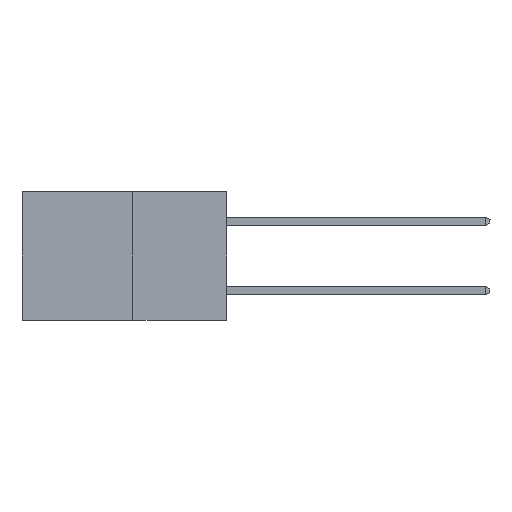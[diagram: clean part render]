
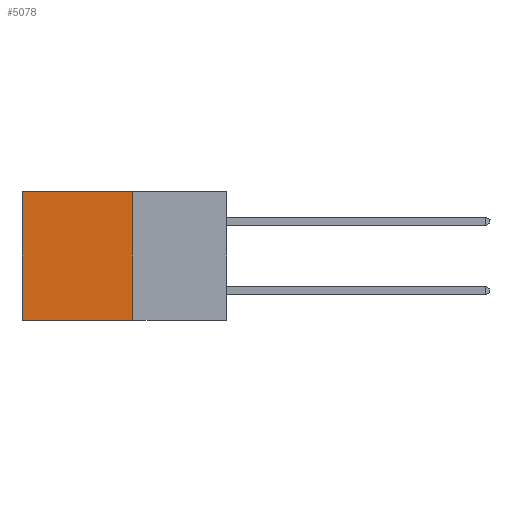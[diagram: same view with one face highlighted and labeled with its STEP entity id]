
A CAD part, left-side view. The second image highlights one B-rep face of the part: STEP entity #5078.
In plain terms, the highlighted planar face has unit normal (-1, 0, 0).
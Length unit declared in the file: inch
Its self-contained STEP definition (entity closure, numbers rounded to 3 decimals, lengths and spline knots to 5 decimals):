
#123 = ORIENTED_EDGE ( 'NONE', *, *, #6466, .T. ) ;
#441 = LINE ( 'NONE', #17034, #2452 ) ;
#500 = DIRECTION ( 'NONE',  ( 0., 1., 0. ) ) ;
#1087 = CARTESIAN_POINT ( 'NONE',  ( 0.277, 0.27, -0.37 ) ) ;
#1097 = VERTEX_POINT ( 'NONE', #2230 ) ;
#1224 = DIRECTION ( 'NONE',  ( 0., 0., -1. ) ) ;
#1623 = LINE ( 'NONE', #4373, #13090 ) ;
#2230 = CARTESIAN_POINT ( 'NONE',  ( 0.277, 0.59, -0.37 ) ) ;
#2452 = VECTOR ( 'NONE', #500, 39.37008 ) ;
#3029 = LINE ( 'NONE', #14663, #14517 ) ;
#4357 = VERTEX_POINT ( 'NONE', #1087 ) ;
#4373 = CARTESIAN_POINT ( 'NONE',  ( 0.277, 0.59, -0.37 ) ) ;
#5078 = ADVANCED_FACE ( 'NONE', ( #9567 ), #16496, .F. ) ;
#6377 = EDGE_CURVE ( 'NONE', #15414, #4357, #3029, .T. ) ;
#6466 = EDGE_CURVE ( 'NONE', #10629, #1097, #1623, .T. ) ;
#6665 = DIRECTION ( 'NONE',  ( 0., 1., 0. ) ) ;
#6745 = EDGE_CURVE ( 'NONE', #15414, #10629, #441, .T. ) ;
#7455 = DIRECTION ( 'NONE',  ( 1., 0., 0. ) ) ;
#8330 = ORIENTED_EDGE ( 'NONE', *, *, #6745, .T. ) ;
#9392 = LINE ( 'NONE', #12560, #12971 ) ;
#9567 = FACE_OUTER_BOUND ( 'NONE', #13771, .T. ) ;
#10029 = EDGE_CURVE ( 'NONE', #4357, #1097, #9392, .T. ) ;
#10629 = VERTEX_POINT ( 'NONE', #13366 ) ;
#12560 = CARTESIAN_POINT ( 'NONE',  ( 0.277, 0.27, -0.37 ) ) ;
#12971 = VECTOR ( 'NONE', #6665, 39.37008 ) ;
#13090 = VECTOR ( 'NONE', #17882, 39.37008 ) ;
#13366 = CARTESIAN_POINT ( 'NONE',  ( 0.277, 0.59, 0. ) ) ;
#13771 = EDGE_LOOP ( 'NONE', ( #123, #17218, #16636, #8330 ) ) ;
#14517 = VECTOR ( 'NONE', #1224, 39.37008 ) ;
#14663 = CARTESIAN_POINT ( 'NONE',  ( 0.277, 0.27, -0.37 ) ) ;
#15414 = VERTEX_POINT ( 'NONE', #18244 ) ;
#15430 = AXIS2_PLACEMENT_3D ( 'NONE', #17933, #7455, #17999 ) ;
#16496 = PLANE ( 'NONE',  #15430 ) ;
#16636 = ORIENTED_EDGE ( 'NONE', *, *, #6377, .F. ) ;
#17034 = CARTESIAN_POINT ( 'NONE',  ( 0.277, 0.27, 0. ) ) ;
#17218 = ORIENTED_EDGE ( 'NONE', *, *, #10029, .F. ) ;
#17882 = DIRECTION ( 'NONE',  ( 0., 0., -1. ) ) ;
#17933 = CARTESIAN_POINT ( 'NONE',  ( 0.277, 0.27, -0.37 ) ) ;
#17999 = DIRECTION ( 'NONE',  ( 0., 0., -1. ) ) ;
#18244 = CARTESIAN_POINT ( 'NONE',  ( 0.277, 0.27, 0. ) ) ;
